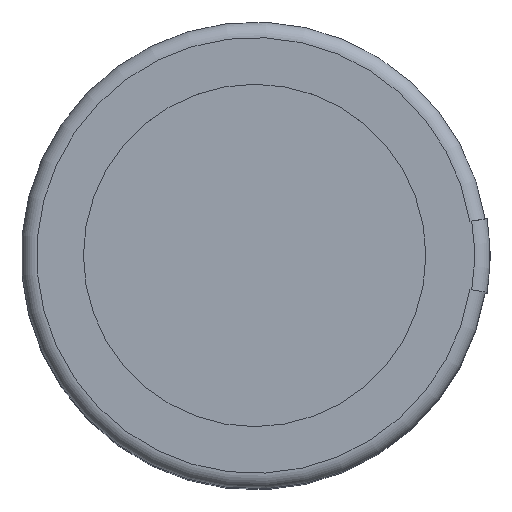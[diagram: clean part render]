
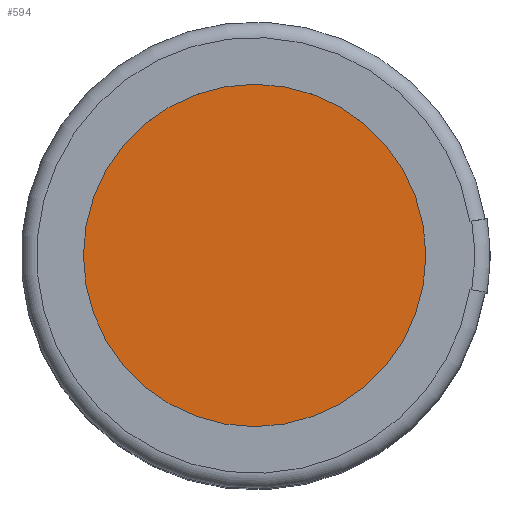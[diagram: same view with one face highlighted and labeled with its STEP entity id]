
A CAD part, top view. The second image highlights one B-rep face of the part: STEP entity #594.
In plain terms, the highlighted planar face has unit normal (0, 0, 1).
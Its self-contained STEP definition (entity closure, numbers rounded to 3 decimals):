
#31=PLANE('',#640);
#49=FACE_OUTER_BOUND('',#83,.T.);
#83=EDGE_LOOP('',(#396,#397));
#185=CIRCLE('',#636,1.833);
#188=CIRCLE('',#639,1.833);
#239=VERTEX_POINT('',#942);
#240=VERTEX_POINT('',#943);
#299=EDGE_CURVE('',#239,#240,#185,.T.);
#303=EDGE_CURVE('',#240,#239,#188,.T.);
#396=ORIENTED_EDGE('',*,*,#299,.F.);
#397=ORIENTED_EDGE('',*,*,#303,.F.);
#594=ADVANCED_FACE('',(#49),#31,.F.);
#636=AXIS2_PLACEMENT_3D('',#944,#739,#740);
#639=AXIS2_PLACEMENT_3D('',#950,#746,#747);
#640=AXIS2_PLACEMENT_3D('',#951,#748,#749);
#739=DIRECTION('center_axis',(0.,0.,-1.));
#740=DIRECTION('ref_axis',(1.,0.,0.));
#746=DIRECTION('center_axis',(0.,0.,-1.));
#747=DIRECTION('ref_axis',(1.,0.,0.));
#748=DIRECTION('center_axis',(0.,0.,-1.));
#749=DIRECTION('ref_axis',(-1.,0.,0.));
#942=CARTESIAN_POINT('',(1.833,0.,6.9));
#943=CARTESIAN_POINT('',(-1.833,0.,6.9));
#944=CARTESIAN_POINT('Origin',(0.,0.,6.9));
#950=CARTESIAN_POINT('Origin',(0.,0.,6.9));
#951=CARTESIAN_POINT('Origin',(0.,0.,6.9));
